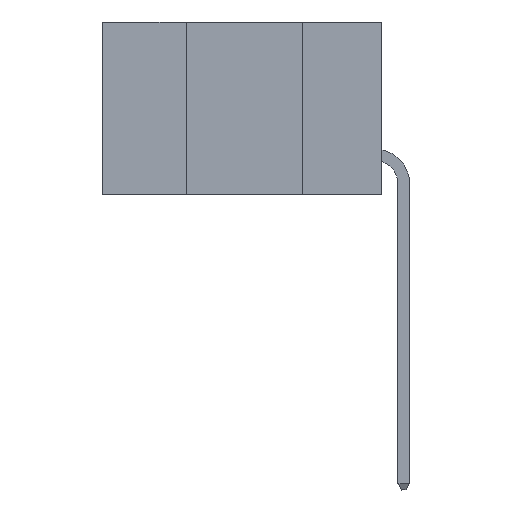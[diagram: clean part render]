
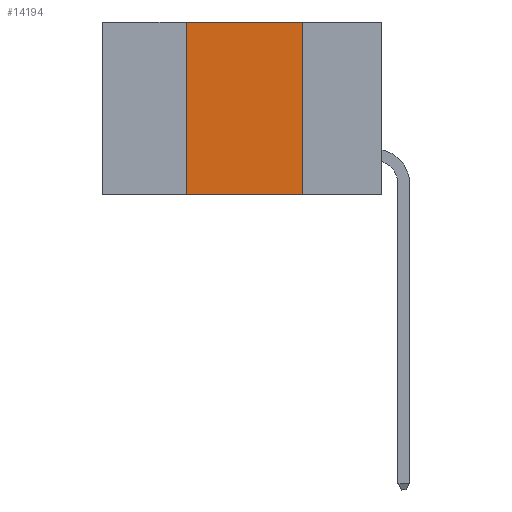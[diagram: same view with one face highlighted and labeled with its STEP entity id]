
A CAD part, left-side view. The second image highlights one B-rep face of the part: STEP entity #14194.
In plain terms, the highlighted planar face has unit normal (-1, 0, 0).
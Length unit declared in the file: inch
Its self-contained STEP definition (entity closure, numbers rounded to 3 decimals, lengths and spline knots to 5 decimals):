
#198 = EDGE_CURVE ( 'NONE', #8346, #20389, #21271, .T. ) ;
#251 = CARTESIAN_POINT ( 'NONE',  ( 0., 0.17, -0.37 ) ) ;
#897 = LINE ( 'NONE', #17934, #5663 ) ;
#1000 = EDGE_CURVE ( 'NONE', #6618, #14331, #8517, .T. ) ;
#2580 = DIRECTION ( 'NONE',  ( 0., -1., 0. ) ) ;
#2840 = DIRECTION ( 'NONE',  ( 0., 0., -1. ) ) ;
#3762 = VECTOR ( 'NONE', #4242, 39.37008 ) ;
#4039 = VECTOR ( 'NONE', #19491, 39.37008 ) ;
#4116 = EDGE_CURVE ( 'NONE', #6618, #8346, #20154, .T. ) ;
#4242 = DIRECTION ( 'NONE',  ( 0., 0., 1. ) ) ;
#4939 = DIRECTION ( 'NONE',  ( 0., 0., -1. ) ) ;
#5663 = VECTOR ( 'NONE', #4939, 39.37008 ) ;
#5673 = CARTESIAN_POINT ( 'NONE',  ( 0., 0.17, 0. ) ) ;
#5996 = ORIENTED_EDGE ( 'NONE', *, *, #4116, .F. ) ;
#6395 = CARTESIAN_POINT ( 'NONE',  ( 0., 0.42, 0. ) ) ;
#6618 = VERTEX_POINT ( 'NONE', #7348 ) ;
#7287 = AXIS2_PLACEMENT_3D ( 'NONE', #17963, #14717, #2840 ) ;
#7348 = CARTESIAN_POINT ( 'NONE',  ( 0., 0.42, -0.37 ) ) ;
#7671 = CARTESIAN_POINT ( 'NONE',  ( 0., 0.6, 0. ) ) ;
#7910 = EDGE_LOOP ( 'NONE', ( #11040, #15244, #5996, #15339 ) ) ;
#8003 = FACE_OUTER_BOUND ( 'NONE', #7910, .T. ) ;
#8346 = VERTEX_POINT ( 'NONE', #6395 ) ;
#8517 = LINE ( 'NONE', #12234, #4039 ) ;
#11040 = ORIENTED_EDGE ( 'NONE', *, *, #11931, .F. ) ;
#11931 = EDGE_CURVE ( 'NONE', #20389, #14331, #897, .T. ) ;
#12234 = CARTESIAN_POINT ( 'NONE',  ( 0., 0.6, -0.37 ) ) ;
#13225 = PLANE ( 'NONE',  #7287 ) ;
#14194 = ADVANCED_FACE ( 'NONE', ( #8003 ), #13225, .F. ) ;
#14331 = VERTEX_POINT ( 'NONE', #251 ) ;
#14634 = CARTESIAN_POINT ( 'NONE',  ( 0., 0.42, 0. ) ) ;
#14717 = DIRECTION ( 'NONE',  ( 1., 0., 0. ) ) ;
#15244 = ORIENTED_EDGE ( 'NONE', *, *, #198, .F. ) ;
#15339 = ORIENTED_EDGE ( 'NONE', *, *, #1000, .T. ) ;
#16477 = VECTOR ( 'NONE', #2580, 39.37008 ) ;
#17934 = CARTESIAN_POINT ( 'NONE',  ( 0., 0.17, 0. ) ) ;
#17963 = CARTESIAN_POINT ( 'NONE',  ( 0., 0.6, 0. ) ) ;
#19491 = DIRECTION ( 'NONE',  ( 0., -1., 0. ) ) ;
#20154 = LINE ( 'NONE', #14634, #3762 ) ;
#20389 = VERTEX_POINT ( 'NONE', #5673 ) ;
#21271 = LINE ( 'NONE', #7671, #16477 ) ;
